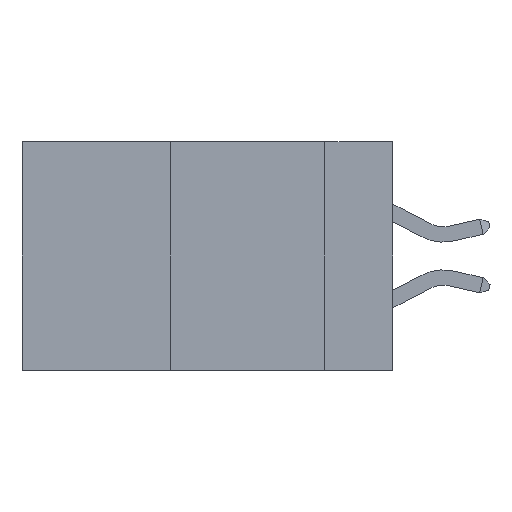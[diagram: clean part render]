
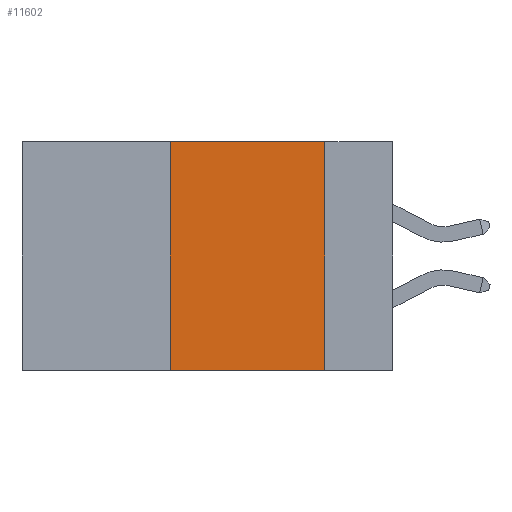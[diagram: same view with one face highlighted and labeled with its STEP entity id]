
A CAD part, left-side view. The second image highlights one B-rep face of the part: STEP entity #11602.
In plain terms, the highlighted planar face has unit normal (-1, 0, 0).
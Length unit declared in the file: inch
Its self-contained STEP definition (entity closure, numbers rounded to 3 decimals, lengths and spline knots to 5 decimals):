
#191 = LINE ( 'NONE', #5210, #7902 ) ;
#393 = CARTESIAN_POINT ( 'NONE',  ( 0., 0.36, 0. ) ) ;
#1545 = EDGE_LOOP ( 'NONE', ( #12219, #3654, #3386, #10277 ) ) ;
#1860 = CARTESIAN_POINT ( 'NONE',  ( 0., 0.6, 0. ) ) ;
#2277 = LINE ( 'NONE', #8030, #10161 ) ;
#2822 = LINE ( 'NONE', #4299, #10432 ) ;
#3058 = EDGE_CURVE ( 'NONE', #7217, #3513, #2822, .T. ) ;
#3386 = ORIENTED_EDGE ( 'NONE', *, *, #8311, .F. ) ;
#3513 = VERTEX_POINT ( 'NONE', #6782 ) ;
#3654 = ORIENTED_EDGE ( 'NONE', *, *, #8373, .F. ) ;
#4096 = VECTOR ( 'NONE', #6796, 39.37008 ) ;
#4299 = CARTESIAN_POINT ( 'NONE',  ( 0., 0.6, -0.37 ) ) ;
#5210 = CARTESIAN_POINT ( 'NONE',  ( 0., 0.6, 0. ) ) ;
#5517 = AXIS2_PLACEMENT_3D ( 'NONE', #1860, #9645, #10585 ) ;
#6121 = VERTEX_POINT ( 'NONE', #393 ) ;
#6782 = CARTESIAN_POINT ( 'NONE',  ( 0., 0.11, -0.37 ) ) ;
#6796 = DIRECTION ( 'NONE',  ( 0., 0., 1. ) ) ;
#7120 = LINE ( 'NONE', #10643, #4096 ) ;
#7217 = VERTEX_POINT ( 'NONE', #9214 ) ;
#7668 = PLANE ( 'NONE',  #5517 ) ;
#7902 = VECTOR ( 'NONE', #10063, 39.37008 ) ;
#8030 = CARTESIAN_POINT ( 'NONE',  ( 0., 0.11, 0. ) ) ;
#8311 = EDGE_CURVE ( 'NONE', #7217, #6121, #7120, .T. ) ;
#8373 = EDGE_CURVE ( 'NONE', #6121, #10435, #191, .T. ) ;
#8681 = CARTESIAN_POINT ( 'NONE',  ( 0., 0.11, 0. ) ) ;
#8991 = EDGE_CURVE ( 'NONE', #10435, #3513, #2277, .T. ) ;
#9214 = CARTESIAN_POINT ( 'NONE',  ( 0., 0.36, -0.37 ) ) ;
#9302 = DIRECTION ( 'NONE',  ( 0., 0., -1. ) ) ;
#9645 = DIRECTION ( 'NONE',  ( 1., 0., 0. ) ) ;
#10063 = DIRECTION ( 'NONE',  ( 0., -1., 0. ) ) ;
#10161 = VECTOR ( 'NONE', #9302, 39.37008 ) ;
#10277 = ORIENTED_EDGE ( 'NONE', *, *, #3058, .T. ) ;
#10432 = VECTOR ( 'NONE', #12283, 39.37008 ) ;
#10435 = VERTEX_POINT ( 'NONE', #8681 ) ;
#10585 = DIRECTION ( 'NONE',  ( 0., 0., -1. ) ) ;
#10643 = CARTESIAN_POINT ( 'NONE',  ( 0., 0.36, 0. ) ) ;
#11511 = FACE_OUTER_BOUND ( 'NONE', #1545, .T. ) ;
#11602 = ADVANCED_FACE ( 'NONE', ( #11511 ), #7668, .F. ) ;
#12219 = ORIENTED_EDGE ( 'NONE', *, *, #8991, .F. ) ;
#12283 = DIRECTION ( 'NONE',  ( 0., -1., 0. ) ) ;
